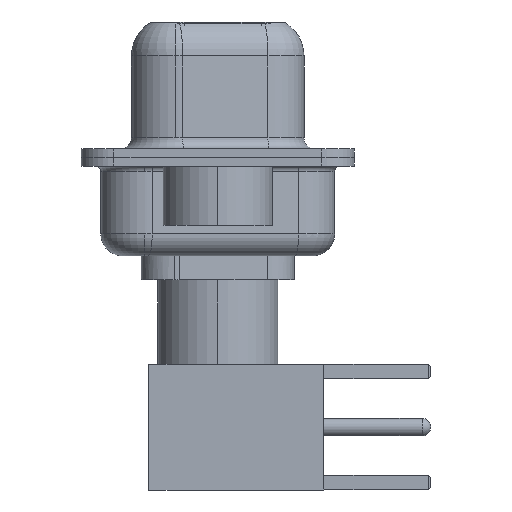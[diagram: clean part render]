
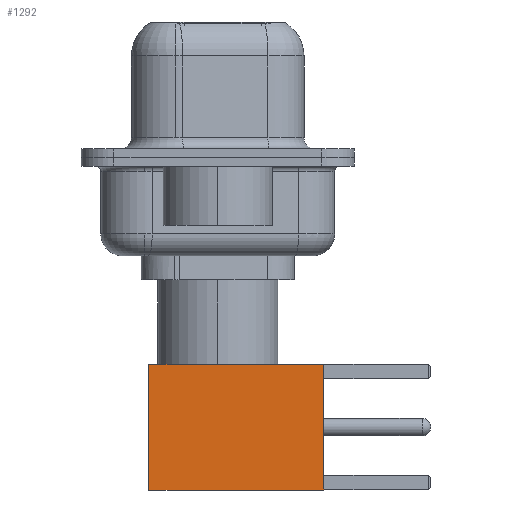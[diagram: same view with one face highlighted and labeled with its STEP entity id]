
A CAD part, left-side view. The second image highlights one B-rep face of the part: STEP entity #1292.
In plain terms, the highlighted face is planar.
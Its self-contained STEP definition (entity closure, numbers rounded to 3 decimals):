
#1260 = VERTEX_POINT ( 'NONE', #14215 ) ;
#1292 = ADVANCED_FACE ( 'NONE', ( #4906 ), #9879, .T. ) ;
#2095 = VERTEX_POINT ( 'NONE', #3829 ) ;
#2219 = LINE ( 'NONE', #11737, #14576 ) ;
#2400 = CARTESIAN_POINT ( 'NONE',  ( -2.875, 2.875, 0. ) ) ;
#2981 = CARTESIAN_POINT ( 'NONE',  ( 0., 2.875, 8. ) ) ;
#3017 = LINE ( 'NONE', #11427, #11256 ) ;
#3829 = CARTESIAN_POINT ( 'NONE',  ( -2.875, 2.875, 0. ) ) ;
#4050 = DIRECTION ( 'NONE',  ( 0., 1., 0. ) ) ;
#4790 = EDGE_CURVE ( 'NONE', #1260, #6664, #2219, .T. ) ;
#4866 = ORIENTED_EDGE ( 'NONE', *, *, #4790, .T. ) ;
#4906 = FACE_OUTER_BOUND ( 'NONE', #13703, .T. ) ;
#4966 = AXIS2_PLACEMENT_3D ( 'NONE', #13567, #4050, #8852 ) ;
#5541 = CARTESIAN_POINT ( 'NONE',  ( -2.875, 2.875, 8. ) ) ;
#5685 = ORIENTED_EDGE ( 'NONE', *, *, #7120, .F. ) ;
#5806 = CARTESIAN_POINT ( 'NONE',  ( 2.875, 2.875, 0. ) ) ;
#5842 = VECTOR ( 'NONE', #6904, 1000. ) ;
#6664 = VERTEX_POINT ( 'NONE', #5806 ) ;
#6904 = DIRECTION ( 'NONE',  ( 0., 0., -1. ) ) ;
#7120 = EDGE_CURVE ( 'NONE', #1260, #11027, #14836, .T. ) ;
#8405 = ORIENTED_EDGE ( 'NONE', *, *, #8600, .F. ) ;
#8600 = EDGE_CURVE ( 'NONE', #11027, #2095, #9565, .T. ) ;
#8852 = DIRECTION ( 'NONE',  ( 0., 0., 1. ) ) ;
#9565 = LINE ( 'NONE', #2400, #5842 ) ;
#9879 = PLANE ( 'NONE',  #4966 ) ;
#10639 = VECTOR ( 'NONE', #11307, 1000. ) ;
#11027 = VERTEX_POINT ( 'NONE', #5541 ) ;
#11256 = VECTOR ( 'NONE', #12605, 1000. ) ;
#11307 = DIRECTION ( 'NONE',  ( -1., 0., 0. ) ) ;
#11427 = CARTESIAN_POINT ( 'NONE',  ( 0., 2.875, 0. ) ) ;
#11737 = CARTESIAN_POINT ( 'NONE',  ( 2.875, 2.875, 0. ) ) ;
#12605 = DIRECTION ( 'NONE',  ( -1., 0., 0. ) ) ;
#13512 = ORIENTED_EDGE ( 'NONE', *, *, #15524, .T. ) ;
#13567 = CARTESIAN_POINT ( 'NONE',  ( 2.875, 2.875, 0. ) ) ;
#13703 = EDGE_LOOP ( 'NONE', ( #4866, #13512, #8405, #5685 ) ) ;
#14215 = CARTESIAN_POINT ( 'NONE',  ( 2.875, 2.875, 8. ) ) ;
#14576 = VECTOR ( 'NONE', #15515, 1000. ) ;
#14836 = LINE ( 'NONE', #2981, #10639 ) ;
#15515 = DIRECTION ( 'NONE',  ( 0., 0., -1. ) ) ;
#15524 = EDGE_CURVE ( 'NONE', #6664, #2095, #3017, .T. ) ;
